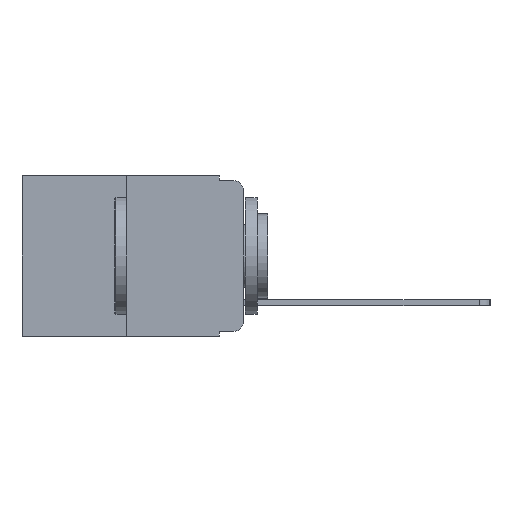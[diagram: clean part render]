
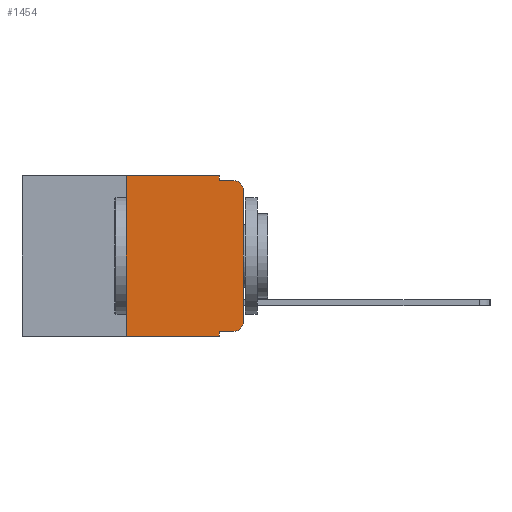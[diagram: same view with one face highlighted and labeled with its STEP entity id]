
A CAD part, left-side view. The second image highlights one B-rep face of the part: STEP entity #1454.
In plain terms, the highlighted planar face has unit normal (-1, 0, 0).
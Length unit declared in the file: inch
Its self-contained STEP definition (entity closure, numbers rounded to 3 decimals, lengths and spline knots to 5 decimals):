
#244 = VECTOR ( 'NONE', #10585, 39.37008 ) ;
#349 = FACE_OUTER_BOUND ( 'NONE', #6110, .T. ) ;
#852 = ORIENTED_EDGE ( 'NONE', *, *, #15574, .T. ) ;
#896 = VERTEX_POINT ( 'NONE', #19418 ) ;
#1091 = EDGE_CURVE ( 'NONE', #3432, #2827, #16548, .T. ) ;
#1143 = CARTESIAN_POINT ( 'NONE',  ( 0., 0.051, 0. ) ) ;
#1454 = ADVANCED_FACE ( 'NONE', ( #349 ), #3888, .F. ) ;
#1740 = ORIENTED_EDGE ( 'NONE', *, *, #10394, .T. ) ;
#2398 = LINE ( 'NONE', #8684, #18796 ) ;
#2827 = VERTEX_POINT ( 'NONE', #5787 ) ;
#2954 = ORIENTED_EDGE ( 'NONE', *, *, #1091, .F. ) ;
#3301 = DIRECTION ( 'NONE',  ( 0., -1., 0. ) ) ;
#3354 = VERTEX_POINT ( 'NONE', #14549 ) ;
#3432 = VERTEX_POINT ( 'NONE', #16312 ) ;
#3685 = CARTESIAN_POINT ( 'NONE',  ( 0., 0.473, 0. ) ) ;
#3745 = CIRCLE ( 'NONE', #16591, 0.02 ) ;
#3888 = PLANE ( 'NONE',  #13870 ) ;
#4309 = LINE ( 'NONE', #15991, #20406 ) ;
#4337 = EDGE_CURVE ( 'NONE', #3432, #16124, #4309, .T. ) ;
#4420 = CARTESIAN_POINT ( 'NONE',  ( 0., 0.02, -0.03 ) ) ;
#4589 = EDGE_CURVE ( 'NONE', #17450, #6164, #20631, .T. ) ;
#5117 = ORIENTED_EDGE ( 'NONE', *, *, #20252, .T. ) ;
#5278 = VERTEX_POINT ( 'NONE', #18989 ) ;
#5390 = LINE ( 'NONE', #10525, #244 ) ;
#5462 = DIRECTION ( 'NONE',  ( 0., -1., 0. ) ) ;
#5552 = CARTESIAN_POINT ( 'NONE',  ( 0., 0., 0. ) ) ;
#5642 = ORIENTED_EDGE ( 'NONE', *, *, #14162, .T. ) ;
#5666 = AXIS2_PLACEMENT_3D ( 'NONE', #8937, #19646, #10477 ) ;
#5787 = CARTESIAN_POINT ( 'NONE',  ( 0., 0.25, 0. ) ) ;
#5857 = VECTOR ( 'NONE', #15681, 39.37008 ) ;
#6000 = DIRECTION ( 'NONE',  ( 1., 0., 0. ) ) ;
#6099 = DIRECTION ( 'NONE',  ( 0., 0., -1. ) ) ;
#6110 = EDGE_LOOP ( 'NONE', ( #5117, #5642, #18563, #19970, #6960, #2954, #15492, #9954, #852, #1740 ) ) ;
#6164 = VERTEX_POINT ( 'NONE', #15478 ) ;
#6506 = CARTESIAN_POINT ( 'NONE',  ( 0., 0.051, 0. ) ) ;
#6960 = ORIENTED_EDGE ( 'NONE', *, *, #9611, .F. ) ;
#7239 = DIRECTION ( 'NONE',  ( 0., 0., 1. ) ) ;
#7313 = VERTEX_POINT ( 'NONE', #9755 ) ;
#7866 = DIRECTION ( 'NONE',  ( 0., 0., -1. ) ) ;
#8205 = VECTOR ( 'NONE', #13278, 39.37008 ) ;
#8684 = CARTESIAN_POINT ( 'NONE',  ( 0., 0.051, -0.333 ) ) ;
#8937 = CARTESIAN_POINT ( 'NONE',  ( 0., 0.02, -0.313 ) ) ;
#8991 = EDGE_CURVE ( 'NONE', #6164, #7313, #5390, .T. ) ;
#9611 = EDGE_CURVE ( 'NONE', #2827, #17450, #19485, .T. ) ;
#9755 = CARTESIAN_POINT ( 'NONE',  ( 0., 0.02, -0.01 ) ) ;
#9954 = ORIENTED_EDGE ( 'NONE', *, *, #16599, .F. ) ;
#10099 = CARTESIAN_POINT ( 'NONE',  ( 0., 0.051, -0.343 ) ) ;
#10117 = LINE ( 'NONE', #1143, #5857 ) ;
#10394 = EDGE_CURVE ( 'NONE', #3354, #5278, #17132, .T. ) ;
#10477 = DIRECTION ( 'NONE',  ( 0., 0., -1. ) ) ;
#10525 = CARTESIAN_POINT ( 'NONE',  ( 0., 0.051, -0.01 ) ) ;
#10585 = DIRECTION ( 'NONE',  ( 0., -1., 0. ) ) ;
#11539 = VERTEX_POINT ( 'NONE', #13426 ) ;
#11727 = CARTESIAN_POINT ( 'NONE',  ( 0., 0.473, 0. ) ) ;
#12076 = DIRECTION ( 'NONE',  ( 0., 0., -1. ) ) ;
#13278 = DIRECTION ( 'NONE',  ( 0., -1., 0. ) ) ;
#13426 = CARTESIAN_POINT ( 'NONE',  ( 0., 0., -0.03 ) ) ;
#13619 = CARTESIAN_POINT ( 'NONE',  ( 0., 0.051, 0. ) ) ;
#13870 = AXIS2_PLACEMENT_3D ( 'NONE', #3685, #6000, #7866 ) ;
#14120 = VECTOR ( 'NONE', #7239, 39.37008 ) ;
#14162 = EDGE_CURVE ( 'NONE', #11539, #7313, #3745, .T. ) ;
#14549 = CARTESIAN_POINT ( 'NONE',  ( 0., 0.02, -0.333 ) ) ;
#15478 = CARTESIAN_POINT ( 'NONE',  ( 0., 0.051, -0.01 ) ) ;
#15482 = DIRECTION ( 'NONE',  ( -1., 0., 0. ) ) ;
#15492 = ORIENTED_EDGE ( 'NONE', *, *, #4337, .T. ) ;
#15574 = EDGE_CURVE ( 'NONE', #896, #3354, #2398, .T. ) ;
#15681 = DIRECTION ( 'NONE',  ( 0., 0., -1. ) ) ;
#15991 = CARTESIAN_POINT ( 'NONE',  ( 0., 0.473, -0.343 ) ) ;
#16037 = DIRECTION ( 'NONE',  ( 0., 0., 1. ) ) ;
#16124 = VERTEX_POINT ( 'NONE', #10099 ) ;
#16169 = VECTOR ( 'NONE', #12076, 39.37008 ) ;
#16312 = CARTESIAN_POINT ( 'NONE',  ( 0., 0.25, -0.343 ) ) ;
#16548 = LINE ( 'NONE', #17514, #17021 ) ;
#16591 = AXIS2_PLACEMENT_3D ( 'NONE', #4420, #15482, #6099 ) ;
#16599 = EDGE_CURVE ( 'NONE', #896, #16124, #10117, .T. ) ;
#17021 = VECTOR ( 'NONE', #16037, 39.37008 ) ;
#17132 = CIRCLE ( 'NONE', #5666, 0.02 ) ;
#17450 = VERTEX_POINT ( 'NONE', #6506 ) ;
#17514 = CARTESIAN_POINT ( 'NONE',  ( 0., 0.25, 0. ) ) ;
#18167 = LINE ( 'NONE', #5552, #14120 ) ;
#18563 = ORIENTED_EDGE ( 'NONE', *, *, #8991, .F. ) ;
#18796 = VECTOR ( 'NONE', #5462, 39.37008 ) ;
#18989 = CARTESIAN_POINT ( 'NONE',  ( 0., 0., -0.313 ) ) ;
#19418 = CARTESIAN_POINT ( 'NONE',  ( 0., 0.051, -0.333 ) ) ;
#19485 = LINE ( 'NONE', #11727, #8205 ) ;
#19646 = DIRECTION ( 'NONE',  ( -1., 0., 0. ) ) ;
#19970 = ORIENTED_EDGE ( 'NONE', *, *, #4589, .F. ) ;
#20252 = EDGE_CURVE ( 'NONE', #5278, #11539, #18167, .T. ) ;
#20406 = VECTOR ( 'NONE', #3301, 39.37008 ) ;
#20631 = LINE ( 'NONE', #13619, #16169 ) ;
